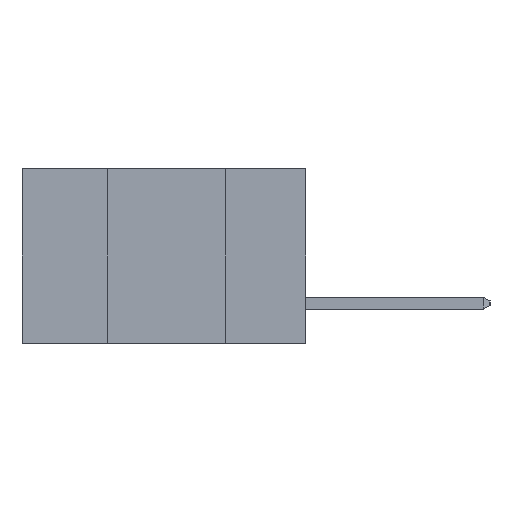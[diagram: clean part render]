
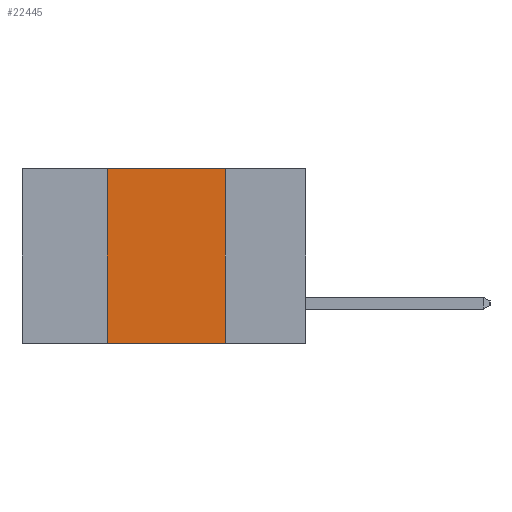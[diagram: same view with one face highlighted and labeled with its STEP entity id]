
A CAD part, left-side view. The second image highlights one B-rep face of the part: STEP entity #22445.
In plain terms, the highlighted planar face has unit normal (-1, 0, 0).
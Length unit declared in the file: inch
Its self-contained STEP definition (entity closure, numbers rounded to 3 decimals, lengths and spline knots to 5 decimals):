
#142 = LINE ( 'NONE', #4079, #11043 ) ;
#1188 = EDGE_LOOP ( 'NONE', ( #1947, #12821, #5320, #2096 ) ) ;
#1947 = ORIENTED_EDGE ( 'NONE', *, *, #2255, .F. ) ;
#2096 = ORIENTED_EDGE ( 'NONE', *, *, #21505, .T. ) ;
#2255 = EDGE_CURVE ( 'NONE', #5806, #8298, #22974, .T. ) ;
#2289 = EDGE_CURVE ( 'NONE', #20778, #23858, #142, .T. ) ;
#2771 = CARTESIAN_POINT ( 'NONE',  ( 0., 0.6, 0. ) ) ;
#4079 = CARTESIAN_POINT ( 'NONE',  ( 0., 0.42, 0. ) ) ;
#5320 = ORIENTED_EDGE ( 'NONE', *, *, #2289, .F. ) ;
#5806 = VERTEX_POINT ( 'NONE', #23614 ) ;
#5928 = VECTOR ( 'NONE', #13060, 39.37008 ) ;
#6041 = LINE ( 'NONE', #12794, #23087 ) ;
#6206 = LINE ( 'NONE', #10070, #16990 ) ;
#6672 = EDGE_CURVE ( 'NONE', #23858, #5806, #6206, .T. ) ;
#8298 = VERTEX_POINT ( 'NONE', #17984 ) ;
#9408 = DIRECTION ( 'NONE',  ( 1., 0., 0. ) ) ;
#9610 = AXIS2_PLACEMENT_3D ( 'NONE', #2771, #9408, #24251 ) ;
#9635 = DIRECTION ( 'NONE',  ( 0., -1., 0. ) ) ;
#10070 = CARTESIAN_POINT ( 'NONE',  ( 0., 0.6, 0. ) ) ;
#11043 = VECTOR ( 'NONE', #22257, 39.37008 ) ;
#11516 = PLANE ( 'NONE',  #9610 ) ;
#12794 = CARTESIAN_POINT ( 'NONE',  ( 0., 0.6, -0.37 ) ) ;
#12821 = ORIENTED_EDGE ( 'NONE', *, *, #6672, .F. ) ;
#13060 = DIRECTION ( 'NONE',  ( 0., 0., -1. ) ) ;
#15982 = FACE_OUTER_BOUND ( 'NONE', #1188, .T. ) ;
#16990 = VECTOR ( 'NONE', #9635, 39.37008 ) ;
#17405 = CARTESIAN_POINT ( 'NONE',  ( 0., 0.17, 0. ) ) ;
#17984 = CARTESIAN_POINT ( 'NONE',  ( 0., 0.17, -0.37 ) ) ;
#18868 = CARTESIAN_POINT ( 'NONE',  ( 0., 0.42, 0. ) ) ;
#19718 = CARTESIAN_POINT ( 'NONE',  ( 0., 0.42, -0.37 ) ) ;
#20778 = VERTEX_POINT ( 'NONE', #19718 ) ;
#21505 = EDGE_CURVE ( 'NONE', #20778, #8298, #6041, .T. ) ;
#22257 = DIRECTION ( 'NONE',  ( 0., 0., 1. ) ) ;
#22445 = ADVANCED_FACE ( 'NONE', ( #15982 ), #11516, .F. ) ;
#22974 = LINE ( 'NONE', #17405, #5928 ) ;
#23087 = VECTOR ( 'NONE', #25377, 39.37008 ) ;
#23614 = CARTESIAN_POINT ( 'NONE',  ( 0., 0.17, 0. ) ) ;
#23858 = VERTEX_POINT ( 'NONE', #18868 ) ;
#24251 = DIRECTION ( 'NONE',  ( 0., 0., -1. ) ) ;
#25377 = DIRECTION ( 'NONE',  ( 0., -1., 0. ) ) ;
